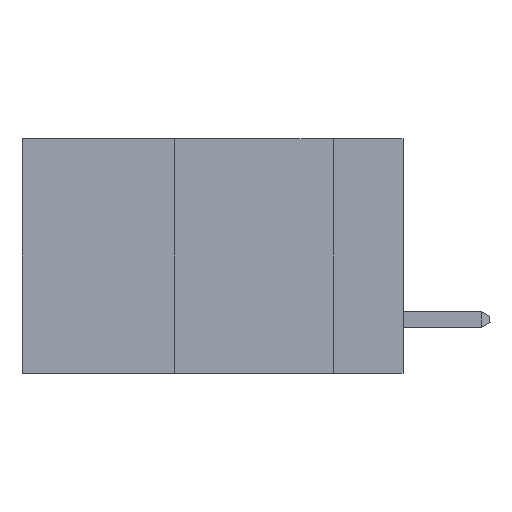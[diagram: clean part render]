
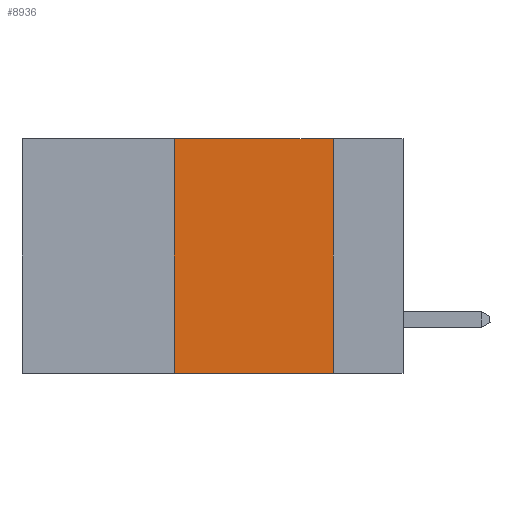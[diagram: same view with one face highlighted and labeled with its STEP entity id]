
A CAD part, left-side view. The second image highlights one B-rep face of the part: STEP entity #8936.
In plain terms, the highlighted planar face has unit normal (-1, 0, 0).
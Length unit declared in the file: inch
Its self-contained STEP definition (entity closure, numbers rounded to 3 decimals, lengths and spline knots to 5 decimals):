
#623 = CARTESIAN_POINT ( 'NONE',  ( 0., 0.6, 0. ) ) ;
#814 = CARTESIAN_POINT ( 'NONE',  ( 0., 0.6, 0. ) ) ;
#933 = CARTESIAN_POINT ( 'NONE',  ( 0., 0.6, -0.37 ) ) ;
#1149 = EDGE_CURVE ( 'NONE', #10973, #9810, #4651, .T. ) ;
#2715 = VECTOR ( 'NONE', #9907, 39.37008 ) ;
#3026 = LINE ( 'NONE', #8443, #5308 ) ;
#4233 = VERTEX_POINT ( 'NONE', #6098 ) ;
#4498 = AXIS2_PLACEMENT_3D ( 'NONE', #623, #16838, #9022 ) ;
#4609 = VECTOR ( 'NONE', #12986, 39.37008 ) ;
#4651 = LINE ( 'NONE', #933, #13655 ) ;
#5308 = VECTOR ( 'NONE', #8558, 39.37008 ) ;
#6098 = CARTESIAN_POINT ( 'NONE',  ( 0., 0.36, 0. ) ) ;
#6118 = DIRECTION ( 'NONE',  ( 0., -1., 0. ) ) ;
#6835 = LINE ( 'NONE', #814, #2715 ) ;
#8443 = CARTESIAN_POINT ( 'NONE',  ( 0., 0.11, 0. ) ) ;
#8558 = DIRECTION ( 'NONE',  ( 0., 0., -1. ) ) ;
#8936 = ADVANCED_FACE ( 'NONE', ( #10398 ), #14954, .F. ) ;
#9022 = DIRECTION ( 'NONE',  ( 0., 0., -1. ) ) ;
#9441 = ORIENTED_EDGE ( 'NONE', *, *, #1149, .T. ) ;
#9597 = EDGE_CURVE ( 'NONE', #12762, #9810, #3026, .T. ) ;
#9781 = CARTESIAN_POINT ( 'NONE',  ( 0., 0.11, 0. ) ) ;
#9810 = VERTEX_POINT ( 'NONE', #12882 ) ;
#9907 = DIRECTION ( 'NONE',  ( 0., -1., 0. ) ) ;
#10131 = LINE ( 'NONE', #16762, #4609 ) ;
#10398 = FACE_OUTER_BOUND ( 'NONE', #12858, .T. ) ;
#10410 = CARTESIAN_POINT ( 'NONE',  ( 0., 0.36, -0.37 ) ) ;
#10786 = ORIENTED_EDGE ( 'NONE', *, *, #9597, .F. ) ;
#10973 = VERTEX_POINT ( 'NONE', #10410 ) ;
#11008 = ORIENTED_EDGE ( 'NONE', *, *, #11560, .F. ) ;
#11560 = EDGE_CURVE ( 'NONE', #10973, #4233, #10131, .T. ) ;
#12304 = ORIENTED_EDGE ( 'NONE', *, *, #13453, .F. ) ;
#12762 = VERTEX_POINT ( 'NONE', #9781 ) ;
#12858 = EDGE_LOOP ( 'NONE', ( #10786, #12304, #11008, #9441 ) ) ;
#12882 = CARTESIAN_POINT ( 'NONE',  ( 0., 0.11, -0.37 ) ) ;
#12986 = DIRECTION ( 'NONE',  ( 0., 0., 1. ) ) ;
#13453 = EDGE_CURVE ( 'NONE', #4233, #12762, #6835, .T. ) ;
#13655 = VECTOR ( 'NONE', #6118, 39.37008 ) ;
#14954 = PLANE ( 'NONE',  #4498 ) ;
#16762 = CARTESIAN_POINT ( 'NONE',  ( 0., 0.36, 0. ) ) ;
#16838 = DIRECTION ( 'NONE',  ( 1., 0., 0. ) ) ;
